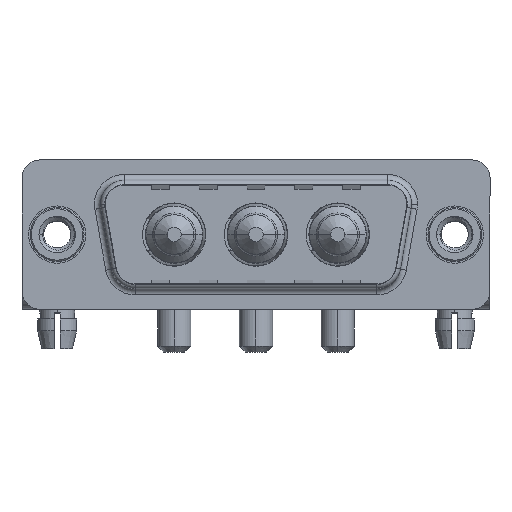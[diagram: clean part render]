
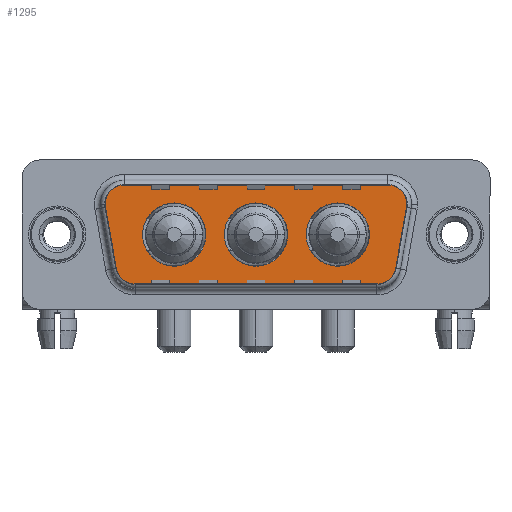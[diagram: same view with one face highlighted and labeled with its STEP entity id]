
A CAD part, top view. The second image highlights one B-rep face of the part: STEP entity #1295.
In plain terms, the highlighted planar face has unit normal (0, 0, 1).
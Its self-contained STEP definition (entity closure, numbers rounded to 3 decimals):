
#25 = CARTESIAN_POINT ( 'NONE',  ( 16.65, 0., 0. ) ) ;
#291 = EDGE_CURVE ( 'NONE', #10454, #2495, #16061, .T. ) ;
#347 = CARTESIAN_POINT ( 'NONE',  ( 6.434, -4.9, 0. ) ) ;
#354 = AXIS2_PLACEMENT_3D ( 'NONE', #16381, #8843, #12732 ) ;
#361 = ORIENTED_EDGE ( 'NONE', *, *, #12649, .F. ) ;
#365 = DIRECTION ( 'NONE',  ( 0., 0., 1. ) ) ;
#787 = EDGE_CURVE ( 'NONE', #8577, #9020, #1742, .T. ) ;
#813 = VERTEX_POINT ( 'NONE', #8418 ) ;
#886 = VECTOR ( 'NONE', #14248, 1000. ) ;
#904 = ORIENTED_EDGE ( 'NONE', *, *, #787, .F. ) ;
#996 = CARTESIAN_POINT ( 'NONE',  ( 20.85, 0., 0. ) ) ;
#1001 = EDGE_CURVE ( 'NONE', #10984, #4858, #6460, .T. ) ;
#1295 = ADVANCED_FACE ( 'NONE', ( #8372, #13432, #10673, #11009 ), #12173, .T. ) ;
#1334 = ORIENTED_EDGE ( 'NONE', *, *, #7241, .T. ) ;
#1361 = EDGE_LOOP ( 'NONE', ( #12641, #6071 ) ) ;
#1588 = DIRECTION ( 'NONE',  ( 1., 0., 0. ) ) ;
#1598 = EDGE_CURVE ( 'NONE', #8061, #10204, #2531, .T. ) ;
#1630 = AXIS2_PLACEMENT_3D ( 'NONE', #9025, #2726, #5218 ) ;
#1733 = EDGE_CURVE ( 'NONE', #2495, #813, #12347, .T. ) ;
#1742 = CIRCLE ( 'NONE', #10487, 2.65 ) ;
#2011 = CARTESIAN_POINT ( 'NONE',  ( 16.65, 0., 0. ) ) ;
#2031 = ORIENTED_EDGE ( 'NONE', *, *, #2099, .T. ) ;
#2041 = CARTESIAN_POINT ( 'NONE',  ( 4.464, -3.247, 0. ) ) ;
#2099 = EDGE_CURVE ( 'NONE', #9929, #3950, #12964, .T. ) ;
#2260 = AXIS2_PLACEMENT_3D ( 'NONE', #14749, #7188, #12345 ) ;
#2273 = CARTESIAN_POINT ( 'NONE',  ( 6.434, -4.9, 0. ) ) ;
#2330 = CARTESIAN_POINT ( 'NONE',  ( 28.836, -3.247, 0. ) ) ;
#2426 = CARTESIAN_POINT ( 'NONE',  ( 9.8, 0., 0. ) ) ;
#2495 = VERTEX_POINT ( 'NONE', #6101 ) ;
#2531 = CIRCLE ( 'NONE', #7840, 2.65 ) ;
#2726 = DIRECTION ( 'NONE',  ( 0., 0., 1. ) ) ;
#2734 = AXIS2_PLACEMENT_3D ( 'NONE', #11542, #14205, #2836 ) ;
#2836 = DIRECTION ( 'NONE',  ( 1., 0., 0. ) ) ;
#2881 = VERTEX_POINT ( 'NONE', #8493 ) ;
#2937 = ORIENTED_EDGE ( 'NONE', *, *, #291, .T. ) ;
#3057 = CARTESIAN_POINT ( 'NONE',  ( 3.441, 2.553, 0. ) ) ;
#3235 = CIRCLE ( 'NONE', #3778, 2. ) ;
#3518 = DIRECTION ( 'NONE',  ( 1., 0., 0. ) ) ;
#3778 = AXIS2_PLACEMENT_3D ( 'NONE', #16079, #9937, #4727 ) ;
#3785 = CIRCLE ( 'NONE', #4849, 2.65 ) ;
#3950 = VERTEX_POINT ( 'NONE', #15620 ) ;
#4165 = EDGE_LOOP ( 'NONE', ( #11162, #361 ) ) ;
#4307 = CIRCLE ( 'NONE', #1630, 2. ) ;
#4325 = ORIENTED_EDGE ( 'NONE', *, *, #1001, .T. ) ;
#4352 = EDGE_CURVE ( 'NONE', #2881, #14790, #3785, .T. ) ;
#4597 = DIRECTION ( 'NONE',  ( 1., 0., 0. ) ) ;
#4727 = DIRECTION ( 'NONE',  ( -1., 0., 0. ) ) ;
#4849 = AXIS2_PLACEMENT_3D ( 'NONE', #2426, #6019, #3518 ) ;
#4858 = VERTEX_POINT ( 'NONE', #2041 ) ;
#5216 = ORIENTED_EDGE ( 'NONE', *, *, #5445, .T. ) ;
#5218 = DIRECTION ( 'NONE',  ( -1., 0., 0. ) ) ;
#5367 = CARTESIAN_POINT ( 'NONE',  ( 5.411, 4.9, 0. ) ) ;
#5445 = EDGE_CURVE ( 'NONE', #13622, #9863, #15732, .T. ) ;
#5452 = DIRECTION ( 'NONE',  ( 0., 0., 1. ) ) ;
#5498 = ORIENTED_EDGE ( 'NONE', *, *, #7018, .F. ) ;
#6019 = DIRECTION ( 'NONE',  ( 0., 0., 1. ) ) ;
#6071 = ORIENTED_EDGE ( 'NONE', *, *, #4352, .F. ) ;
#6101 = CARTESIAN_POINT ( 'NONE',  ( 29.859, 2.553, 0. ) ) ;
#6349 = ORIENTED_EDGE ( 'NONE', *, *, #13272, .T. ) ;
#6460 = LINE ( 'NONE', #3057, #7851 ) ;
#6604 = CARTESIAN_POINT ( 'NONE',  ( 26.15, 0., 0. ) ) ;
#6656 = CIRCLE ( 'NONE', #13007, 2.65 ) ;
#6772 = AXIS2_PLACEMENT_3D ( 'NONE', #7933, #365, #9007 ) ;
#6917 = DIRECTION ( 'NONE',  ( 1., 0., 0. ) ) ;
#7018 = EDGE_CURVE ( 'NONE', #9020, #8577, #8633, .T. ) ;
#7163 = DIRECTION ( 'NONE',  ( 0., 0., 1. ) ) ;
#7188 = DIRECTION ( 'NONE',  ( 0., 0., 1. ) ) ;
#7241 = EDGE_CURVE ( 'NONE', #9863, #10984, #11781, .T. ) ;
#7291 = AXIS2_PLACEMENT_3D ( 'NONE', #8024, #5452, #7862 ) ;
#7433 = VECTOR ( 'NONE', #1588, 1000. ) ;
#7840 = AXIS2_PLACEMENT_3D ( 'NONE', #25, #12502, #15312 ) ;
#7851 = VECTOR ( 'NONE', #14584, 1000. ) ;
#7862 = DIRECTION ( 'NONE',  ( 1., 0., 0. ) ) ;
#7933 = CARTESIAN_POINT ( 'NONE',  ( 27.889, 2.9, 0. ) ) ;
#8024 = CARTESIAN_POINT ( 'NONE',  ( 26.866, -2.9, 0. ) ) ;
#8061 = VERTEX_POINT ( 'NONE', #8235 ) ;
#8235 = CARTESIAN_POINT ( 'NONE',  ( 19.3, 0., 0. ) ) ;
#8289 = DIRECTION ( 'NONE',  ( 1., 0., 0. ) ) ;
#8360 = CARTESIAN_POINT ( 'NONE',  ( 29.859, 2.553, 0. ) ) ;
#8372 = FACE_BOUND ( 'NONE', #4165, .T. ) ;
#8389 = ORIENTED_EDGE ( 'NONE', *, *, #1733, .T. ) ;
#8418 = CARTESIAN_POINT ( 'NONE',  ( 29.889, 2.9, 0. ) ) ;
#8493 = CARTESIAN_POINT ( 'NONE',  ( 7.15, 0., 0. ) ) ;
#8577 = VERTEX_POINT ( 'NONE', #6604 ) ;
#8586 = EDGE_CURVE ( 'NONE', #3950, #10454, #14440, .T. ) ;
#8633 = CIRCLE ( 'NONE', #2260, 2.65 ) ;
#8843 = DIRECTION ( 'NONE',  ( 0., 0., 1. ) ) ;
#9007 = DIRECTION ( 'NONE',  ( -1., 0., 0. ) ) ;
#9020 = VERTEX_POINT ( 'NONE', #996 ) ;
#9025 = CARTESIAN_POINT ( 'NONE',  ( 6.434, -2.9, 0. ) ) ;
#9443 = DIRECTION ( 'NONE',  ( 0., 0., 1. ) ) ;
#9811 = CARTESIAN_POINT ( 'NONE',  ( 23.5, 0., 0. ) ) ;
#9863 = VERTEX_POINT ( 'NONE', #5367 ) ;
#9929 = VERTEX_POINT ( 'NONE', #2273 ) ;
#9937 = DIRECTION ( 'NONE',  ( 0., 0., 1. ) ) ;
#10192 = CARTESIAN_POINT ( 'NONE',  ( 12.45, 0., 0. ) ) ;
#10204 = VERTEX_POINT ( 'NONE', #11792 ) ;
#10333 = CARTESIAN_POINT ( 'NONE',  ( 3.441, 2.553, 0. ) ) ;
#10453 = AXIS2_PLACEMENT_3D ( 'NONE', #10756, #9443, #8289 ) ;
#10454 = VERTEX_POINT ( 'NONE', #2330 ) ;
#10487 = AXIS2_PLACEMENT_3D ( 'NONE', #9811, #7163, #6917 ) ;
#10673 = FACE_BOUND ( 'NONE', #1361, .T. ) ;
#10756 = CARTESIAN_POINT ( 'NONE',  ( 26.866, -2.9, 0. ) ) ;
#10984 = VERTEX_POINT ( 'NONE', #10333 ) ;
#11009 = FACE_OUTER_BOUND ( 'NONE', #13747, .T. ) ;
#11049 = VECTOR ( 'NONE', #15886, 1000. ) ;
#11162 = ORIENTED_EDGE ( 'NONE', *, *, #1598, .F. ) ;
#11542 = CARTESIAN_POINT ( 'NONE',  ( 9.8, 0., 0. ) ) ;
#11781 = CIRCLE ( 'NONE', #354, 2. ) ;
#11792 = CARTESIAN_POINT ( 'NONE',  ( 14., 0., 0. ) ) ;
#12132 = ORIENTED_EDGE ( 'NONE', *, *, #8586, .T. ) ;
#12173 = PLANE ( 'NONE',  #10453 ) ;
#12276 = CIRCLE ( 'NONE', #2734, 2.65 ) ;
#12345 = DIRECTION ( 'NONE',  ( 1., 0., 0. ) ) ;
#12347 = CIRCLE ( 'NONE', #6772, 2. ) ;
#12502 = DIRECTION ( 'NONE',  ( 0., 0., 1. ) ) ;
#12641 = ORIENTED_EDGE ( 'NONE', *, *, #15637, .F. ) ;
#12649 = EDGE_CURVE ( 'NONE', #10204, #8061, #6656, .T. ) ;
#12732 = DIRECTION ( 'NONE',  ( 1., 0., 0. ) ) ;
#12964 = LINE ( 'NONE', #347, #7433 ) ;
#13007 = AXIS2_PLACEMENT_3D ( 'NONE', #2011, #15701, #4597 ) ;
#13272 = EDGE_CURVE ( 'NONE', #4858, #9929, #4307, .T. ) ;
#13432 = FACE_BOUND ( 'NONE', #14786, .T. ) ;
#13622 = VERTEX_POINT ( 'NONE', #13974 ) ;
#13747 = EDGE_LOOP ( 'NONE', ( #12132, #2937, #8389, #14998, #5216, #1334, #4325, #6349, #2031 ) ) ;
#13974 = CARTESIAN_POINT ( 'NONE',  ( 27.889, 4.9, 0. ) ) ;
#14205 = DIRECTION ( 'NONE',  ( 0., 0., 1. ) ) ;
#14248 = DIRECTION ( 'NONE',  ( -1., 0., 0. ) ) ;
#14440 = CIRCLE ( 'NONE', #7291, 2. ) ;
#14584 = DIRECTION ( 'NONE',  ( 0.174, -0.985, 0. ) ) ;
#14749 = CARTESIAN_POINT ( 'NONE',  ( 23.5, 0., 0. ) ) ;
#14786 = EDGE_LOOP ( 'NONE', ( #904, #5498 ) ) ;
#14790 = VERTEX_POINT ( 'NONE', #10192 ) ;
#14998 = ORIENTED_EDGE ( 'NONE', *, *, #15116, .T. ) ;
#15116 = EDGE_CURVE ( 'NONE', #813, #13622, #3235, .T. ) ;
#15312 = DIRECTION ( 'NONE',  ( 1., 0., 0. ) ) ;
#15492 = CARTESIAN_POINT ( 'NONE',  ( 5.411, 4.9, 0. ) ) ;
#15620 = CARTESIAN_POINT ( 'NONE',  ( 26.866, -4.9, 0. ) ) ;
#15637 = EDGE_CURVE ( 'NONE', #14790, #2881, #12276, .T. ) ;
#15701 = DIRECTION ( 'NONE',  ( 0., 0., 1. ) ) ;
#15732 = LINE ( 'NONE', #15492, #886 ) ;
#15886 = DIRECTION ( 'NONE',  ( 0.174, 0.985, 0. ) ) ;
#16061 = LINE ( 'NONE', #8360, #11049 ) ;
#16079 = CARTESIAN_POINT ( 'NONE',  ( 27.889, 2.9, 0. ) ) ;
#16381 = CARTESIAN_POINT ( 'NONE',  ( 5.411, 2.9, 0. ) ) ;
